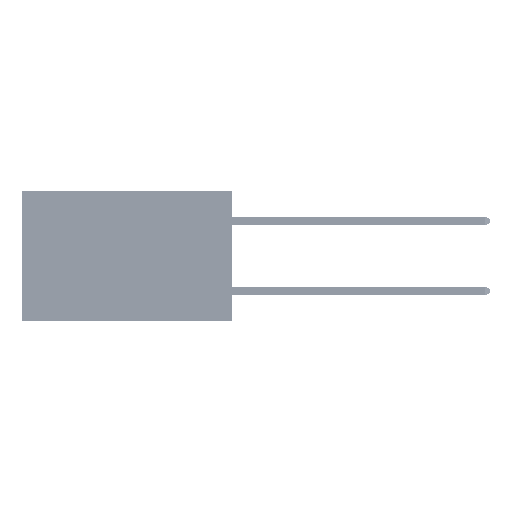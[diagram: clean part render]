
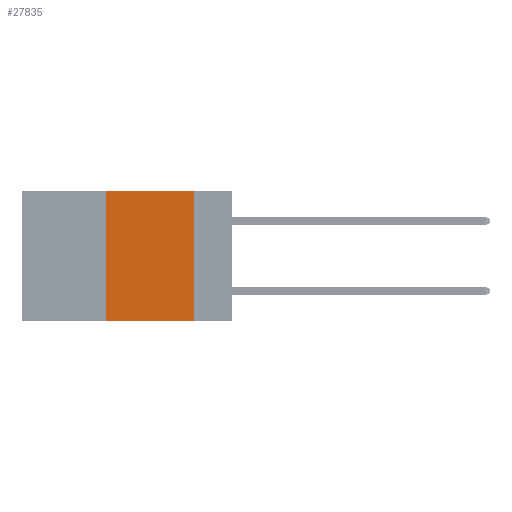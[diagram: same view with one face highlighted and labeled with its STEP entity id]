
A CAD part, left-side view. The second image highlights one B-rep face of the part: STEP entity #27835.
In plain terms, the highlighted planar face has unit normal (-1, 0, 0).
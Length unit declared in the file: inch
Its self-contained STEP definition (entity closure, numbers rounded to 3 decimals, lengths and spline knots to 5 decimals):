
#1446 = CARTESIAN_POINT ( 'NONE',  ( 0., 0.11, -0.37 ) ) ;
#4488 = PLANE ( 'NONE',  #4991 ) ;
#4884 = FACE_OUTER_BOUND ( 'NONE', #24961, .T. ) ;
#4991 = AXIS2_PLACEMENT_3D ( 'NONE', #38992, #46742, #23951 ) ;
#5159 = EDGE_CURVE ( 'NONE', #34033, #32457, #10739, .T. ) ;
#7158 = ORIENTED_EDGE ( 'NONE', *, *, #5159, .F. ) ;
#10739 = LINE ( 'NONE', #27970, #14935 ) ;
#12585 = VECTOR ( 'NONE', #45178, 39.37008 ) ;
#12673 = CARTESIAN_POINT ( 'NONE',  ( 0., 0.36, 0. ) ) ;
#13004 = DIRECTION ( 'NONE',  ( 0., -1., 0. ) ) ;
#14935 = VECTOR ( 'NONE', #31629, 39.37008 ) ;
#15620 = LINE ( 'NONE', #41189, #12585 ) ;
#17430 = EDGE_CURVE ( 'NONE', #34033, #37911, #15620, .T. ) ;
#18342 = DIRECTION ( 'NONE',  ( 0., 0., -1. ) ) ;
#20041 = LINE ( 'NONE', #24831, #42482 ) ;
#20410 = LINE ( 'NONE', #44810, #25743 ) ;
#23951 = DIRECTION ( 'NONE',  ( 0., 0., -1. ) ) ;
#24831 = CARTESIAN_POINT ( 'NONE',  ( 0., 0.6, 0. ) ) ;
#24961 = EDGE_LOOP ( 'NONE', ( #43292, #47363, #7158, #33807 ) ) ;
#25631 = VERTEX_POINT ( 'NONE', #28296 ) ;
#25743 = VECTOR ( 'NONE', #18342, 39.37008 ) ;
#26473 = CARTESIAN_POINT ( 'NONE',  ( 0., 0.36, -0.37 ) ) ;
#27835 = ADVANCED_FACE ( 'NONE', ( #4884 ), #4488, .F. ) ;
#27970 = CARTESIAN_POINT ( 'NONE',  ( 0., 0.36, 0. ) ) ;
#28296 = CARTESIAN_POINT ( 'NONE',  ( 0., 0.11, 0. ) ) ;
#31629 = DIRECTION ( 'NONE',  ( 0., 0., 1. ) ) ;
#32457 = VERTEX_POINT ( 'NONE', #12673 ) ;
#32688 = EDGE_CURVE ( 'NONE', #32457, #25631, #20041, .T. ) ;
#33807 = ORIENTED_EDGE ( 'NONE', *, *, #17430, .T. ) ;
#34033 = VERTEX_POINT ( 'NONE', #26473 ) ;
#37911 = VERTEX_POINT ( 'NONE', #1446 ) ;
#38992 = CARTESIAN_POINT ( 'NONE',  ( 0., 0.6, 0. ) ) ;
#41189 = CARTESIAN_POINT ( 'NONE',  ( 0., 0.6, -0.37 ) ) ;
#42482 = VECTOR ( 'NONE', #13004, 39.37008 ) ;
#43292 = ORIENTED_EDGE ( 'NONE', *, *, #45727, .F. ) ;
#44810 = CARTESIAN_POINT ( 'NONE',  ( 0., 0.11, 0. ) ) ;
#45178 = DIRECTION ( 'NONE',  ( 0., -1., 0. ) ) ;
#45727 = EDGE_CURVE ( 'NONE', #25631, #37911, #20410, .T. ) ;
#46742 = DIRECTION ( 'NONE',  ( 1., 0., 0. ) ) ;
#47363 = ORIENTED_EDGE ( 'NONE', *, *, #32688, .F. ) ;
